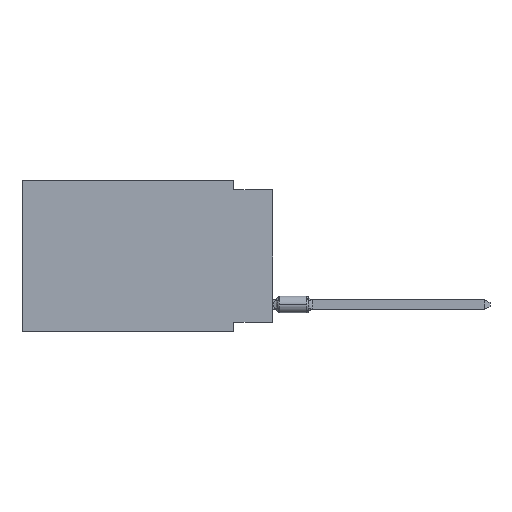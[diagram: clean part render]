
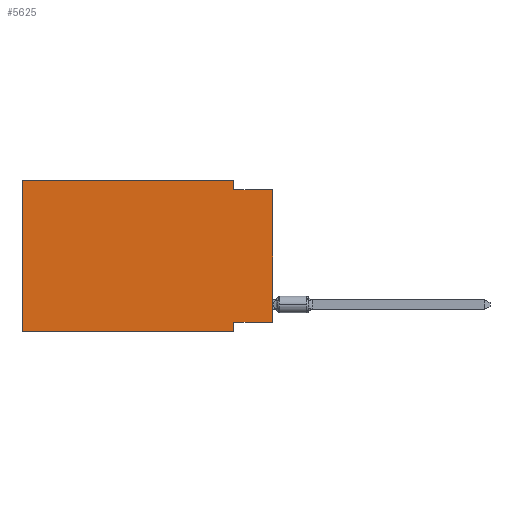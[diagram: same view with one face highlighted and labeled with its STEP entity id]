
A CAD part, left-side view. The second image highlights one B-rep face of the part: STEP entity #5625.
In plain terms, the highlighted planar face has unit normal (-1, 0, 0).
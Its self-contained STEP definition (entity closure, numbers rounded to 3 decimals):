
#401 = VECTOR ( 'NONE', #2526, 1000. ) ;
#551 = CARTESIAN_POINT ( 'NONE',  ( 0., 2.54, -9.906 ) ) ;
#629 = ORIENTED_EDGE ( 'NONE', *, *, #7113, .T. ) ;
#876 = CARTESIAN_POINT ( 'NONE',  ( 0., 2.54, -0.635 ) ) ;
#910 = DIRECTION ( 'NONE',  ( 0., -1., 0. ) ) ;
#1049 = LINE ( 'NONE', #3457, #15387 ) ;
#1103 = LINE ( 'NONE', #3287, #14054 ) ;
#1480 = VERTEX_POINT ( 'NONE', #5747 ) ;
#2329 = CARTESIAN_POINT ( 'NONE',  ( 0., 16.383, 0. ) ) ;
#2526 = DIRECTION ( 'NONE',  ( 0., 1., 0. ) ) ;
#2645 = VERTEX_POINT ( 'NONE', #15173 ) ;
#2814 = DIRECTION ( 'NONE',  ( 0., 0., 1. ) ) ;
#2998 = ORIENTED_EDGE ( 'NONE', *, *, #5326, .F. ) ;
#3287 = CARTESIAN_POINT ( 'NONE',  ( 0., 0., -0.635 ) ) ;
#3337 = EDGE_CURVE ( 'NONE', #1480, #12168, #1049, .T. ) ;
#3420 = DIRECTION ( 'NONE',  ( 0., -1., 0. ) ) ;
#3457 = CARTESIAN_POINT ( 'NONE',  ( 0., 0., 0. ) ) ;
#3819 = DIRECTION ( 'NONE',  ( 0., 0., -1. ) ) ;
#4246 = EDGE_CURVE ( 'NONE', #7392, #5397, #14444, .T. ) ;
#4276 = LINE ( 'NONE', #9077, #6690 ) ;
#4925 = ORIENTED_EDGE ( 'NONE', *, *, #7056, .F. ) ;
#5303 = CARTESIAN_POINT ( 'NONE',  ( 0., 2.54, -9.906 ) ) ;
#5326 = EDGE_CURVE ( 'NONE', #5397, #12168, #1103, .T. ) ;
#5397 = VERTEX_POINT ( 'NONE', #876 ) ;
#5398 = DIRECTION ( 'NONE',  ( 1., 0., 0. ) ) ;
#5625 = ADVANCED_FACE ( 'NONE', ( #10272 ), #13608, .F. ) ;
#5747 = CARTESIAN_POINT ( 'NONE',  ( 0., 0., -9.271 ) ) ;
#5842 = LINE ( 'NONE', #2329, #6672 ) ;
#6586 = CARTESIAN_POINT ( 'NONE',  ( 0., 16.383, -9.906 ) ) ;
#6600 = VERTEX_POINT ( 'NONE', #6586 ) ;
#6672 = VECTOR ( 'NONE', #3420, 1000. ) ;
#6690 = VECTOR ( 'NONE', #2814, 1000. ) ;
#7056 = EDGE_CURVE ( 'NONE', #2645, #10614, #7822, .T. ) ;
#7113 = EDGE_CURVE ( 'NONE', #6600, #10614, #12846, .T. ) ;
#7392 = VERTEX_POINT ( 'NONE', #13246 ) ;
#7696 = DIRECTION ( 'NONE',  ( 0., 0., -1. ) ) ;
#7706 = CARTESIAN_POINT ( 'NONE',  ( 0., 0., -0.635 ) ) ;
#7822 = LINE ( 'NONE', #5303, #7889 ) ;
#7889 = VECTOR ( 'NONE', #10106, 1000. ) ;
#8077 = DIRECTION ( 'NONE',  ( 0., -1., 0. ) ) ;
#8549 = AXIS2_PLACEMENT_3D ( 'NONE', #10054, #5398, #7696 ) ;
#8633 = EDGE_LOOP ( 'NONE', ( #11087, #2998, #14566, #9131, #15422, #629, #4925, #15490 ) ) ;
#9077 = CARTESIAN_POINT ( 'NONE',  ( 0., 16.383, 0. ) ) ;
#9131 = ORIENTED_EDGE ( 'NONE', *, *, #14428, .F. ) ;
#9539 = VERTEX_POINT ( 'NONE', #14657 ) ;
#9860 = VECTOR ( 'NONE', #3819, 1000. ) ;
#9912 = VECTOR ( 'NONE', #910, 1000. ) ;
#9992 = LINE ( 'NONE', #14798, #401 ) ;
#10054 = CARTESIAN_POINT ( 'NONE',  ( 0., 16.383, 0. ) ) ;
#10106 = DIRECTION ( 'NONE',  ( 0., 0., -1. ) ) ;
#10272 = FACE_OUTER_BOUND ( 'NONE', #8633, .T. ) ;
#10473 = CARTESIAN_POINT ( 'NONE',  ( 0., 16.383, -9.906 ) ) ;
#10614 = VERTEX_POINT ( 'NONE', #551 ) ;
#11087 = ORIENTED_EDGE ( 'NONE', *, *, #3337, .T. ) ;
#11911 = CARTESIAN_POINT ( 'NONE',  ( 0., 2.54, 0. ) ) ;
#12168 = VERTEX_POINT ( 'NONE', #7706 ) ;
#12604 = EDGE_CURVE ( 'NONE', #6600, #9539, #4276, .T. ) ;
#12846 = LINE ( 'NONE', #10473, #9912 ) ;
#13071 = DIRECTION ( 'NONE',  ( 0., 0., 1. ) ) ;
#13246 = CARTESIAN_POINT ( 'NONE',  ( 0., 2.54, 0. ) ) ;
#13263 = EDGE_CURVE ( 'NONE', #1480, #2645, #9992, .T. ) ;
#13608 = PLANE ( 'NONE',  #8549 ) ;
#14054 = VECTOR ( 'NONE', #8077, 1000. ) ;
#14428 = EDGE_CURVE ( 'NONE', #9539, #7392, #5842, .T. ) ;
#14444 = LINE ( 'NONE', #11911, #9860 ) ;
#14566 = ORIENTED_EDGE ( 'NONE', *, *, #4246, .F. ) ;
#14657 = CARTESIAN_POINT ( 'NONE',  ( 0., 16.383, 0. ) ) ;
#14798 = CARTESIAN_POINT ( 'NONE',  ( 0., 0., -9.271 ) ) ;
#15173 = CARTESIAN_POINT ( 'NONE',  ( 0., 2.54, -9.271 ) ) ;
#15387 = VECTOR ( 'NONE', #13071, 1000. ) ;
#15422 = ORIENTED_EDGE ( 'NONE', *, *, #12604, .F. ) ;
#15490 = ORIENTED_EDGE ( 'NONE', *, *, #13263, .F. ) ;
